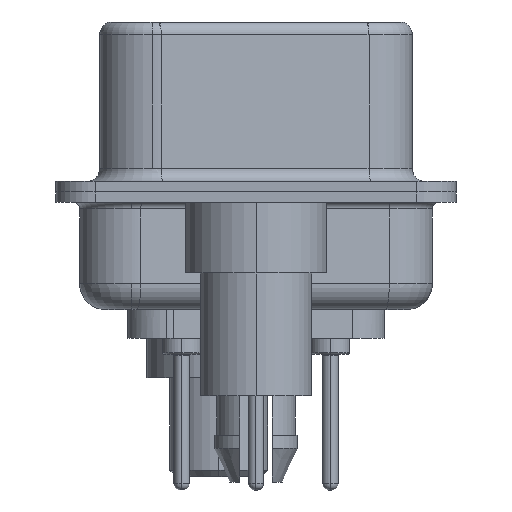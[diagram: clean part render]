
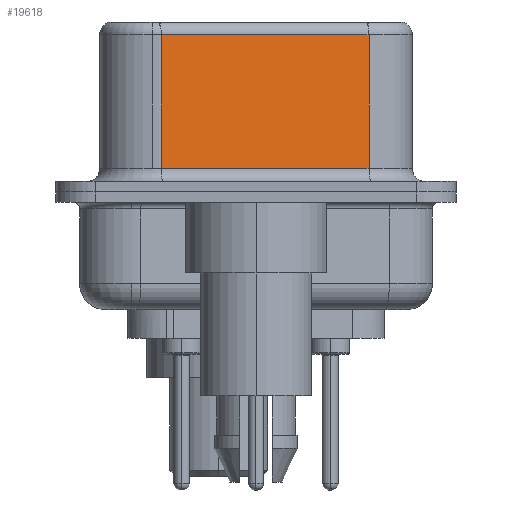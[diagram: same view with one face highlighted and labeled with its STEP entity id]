
A CAD part, left-side view. The second image highlights one B-rep face of the part: STEP entity #19618.
In plain terms, the highlighted planar face has unit normal (-0.985, -0.174, 0).
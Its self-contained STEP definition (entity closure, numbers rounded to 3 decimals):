
#1072 = LINE ( 'NONE', #31881, #3897 ) ;
#2063 = ORIENTED_EDGE ( 'NONE', *, *, #30558, .F. ) ;
#3897 = VECTOR ( 'NONE', #26673, 1000. ) ;
#5326 = DIRECTION ( 'NONE',  ( -0.174, 0.985, 0. ) ) ;
#5866 = CARTESIAN_POINT ( 'NONE',  ( 5.132, -4.322, 0.9 ) ) ;
#6644 = EDGE_LOOP ( 'NONE', ( #2063, #24716, #25586, #8753 ) ) ;
#6811 = DIRECTION ( 'NONE',  ( 0.985, 0.174, 0. ) ) ;
#7235 = AXIS2_PLACEMENT_3D ( 'NONE', #15355, #6811, #5326 ) ;
#8284 = CARTESIAN_POINT ( 'NONE',  ( 5.132, -4.322, 6.02 ) ) ;
#8753 = ORIENTED_EDGE ( 'NONE', *, *, #13023, .T. ) ;
#9093 = VERTEX_POINT ( 'NONE', #25439 ) ;
#12772 = PLANE ( 'NONE',  #7235 ) ;
#13023 = EDGE_CURVE ( 'NONE', #14396, #29140, #26378, .T. ) ;
#14396 = VERTEX_POINT ( 'NONE', #25726 ) ;
#15355 = CARTESIAN_POINT ( 'NONE',  ( 5.132, -4.322, 6.52 ) ) ;
#19179 = VECTOR ( 'NONE', #21380, 1000. ) ;
#19423 = CARTESIAN_POINT ( 'NONE',  ( 5.132, -4.322, 6.02 ) ) ;
#19618 = ADVANCED_FACE ( 'NONE', ( #32248 ), #12772, .F. ) ;
#20394 = VECTOR ( 'NONE', #24889, 1000. ) ;
#21380 = DIRECTION ( 'NONE',  ( 0.174, -0.985, 0. ) ) ;
#21448 = CARTESIAN_POINT ( 'NONE',  ( 5.132, -4.322, 0.9 ) ) ;
#23098 = LINE ( 'NONE', #25195, #29966 ) ;
#24716 = ORIENTED_EDGE ( 'NONE', *, *, #27440, .T. ) ;
#24889 = DIRECTION ( 'NONE',  ( -0.174, 0.985, 0. ) ) ;
#25195 = CARTESIAN_POINT ( 'NONE',  ( 5.132, -4.322, 6.52 ) ) ;
#25439 = CARTESIAN_POINT ( 'NONE',  ( 3.73, 3.628, 6.02 ) ) ;
#25586 = ORIENTED_EDGE ( 'NONE', *, *, #29774, .T. ) ;
#25726 = CARTESIAN_POINT ( 'NONE',  ( 3.73, 3.628, 0.9 ) ) ;
#26378 = LINE ( 'NONE', #5866, #19179 ) ;
#26673 = DIRECTION ( 'NONE',  ( 0., 0., -1. ) ) ;
#27440 = EDGE_CURVE ( 'NONE', #28947, #9093, #32511, .T. ) ;
#27915 = DIRECTION ( 'NONE',  ( 0., 0., -1. ) ) ;
#28947 = VERTEX_POINT ( 'NONE', #8284 ) ;
#29140 = VERTEX_POINT ( 'NONE', #21448 ) ;
#29774 = EDGE_CURVE ( 'NONE', #9093, #14396, #1072, .T. ) ;
#29966 = VECTOR ( 'NONE', #27915, 1000. ) ;
#30558 = EDGE_CURVE ( 'NONE', #28947, #29140, #23098, .T. ) ;
#31881 = CARTESIAN_POINT ( 'NONE',  ( 3.73, 3.628, 6.52 ) ) ;
#32248 = FACE_OUTER_BOUND ( 'NONE', #6644, .T. ) ;
#32511 = LINE ( 'NONE', #19423, #20394 ) ;
